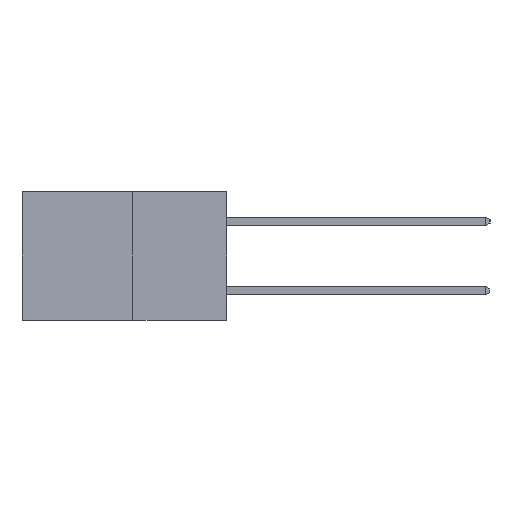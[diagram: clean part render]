
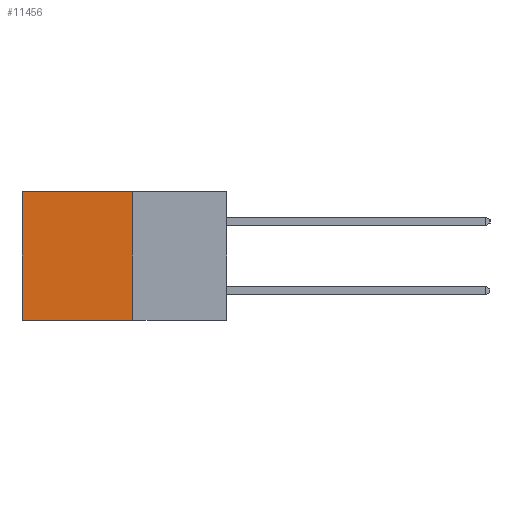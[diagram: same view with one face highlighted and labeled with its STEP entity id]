
A CAD part, left-side view. The second image highlights one B-rep face of the part: STEP entity #11456.
In plain terms, the highlighted planar face has unit normal (-1, 0, 0).
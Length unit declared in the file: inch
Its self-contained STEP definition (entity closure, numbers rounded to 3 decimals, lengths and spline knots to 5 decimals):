
#144 = LINE ( 'NONE', #14034, #7652 ) ;
#267 = EDGE_CURVE ( 'NONE', #5289, #16820, #5860, .T. ) ;
#419 = CARTESIAN_POINT ( 'NONE',  ( 0.277, 0.27, 0. ) ) ;
#1149 = DIRECTION ( 'NONE',  ( 0., 1., 0. ) ) ;
#1166 = CARTESIAN_POINT ( 'NONE',  ( 0.277, 0.27, 0. ) ) ;
#2502 = DIRECTION ( 'NONE',  ( 0., 0., -1. ) ) ;
#2637 = CARTESIAN_POINT ( 'NONE',  ( 0.277, 0.27, -0.37 ) ) ;
#2943 = EDGE_LOOP ( 'NONE', ( #11255, #3657, #3782, #6845 ) ) ;
#3618 = DIRECTION ( 'NONE',  ( 0., 0., -1. ) ) ;
#3657 = ORIENTED_EDGE ( 'NONE', *, *, #11526, .F. ) ;
#3782 = ORIENTED_EDGE ( 'NONE', *, *, #267, .F. ) ;
#4206 = CARTESIAN_POINT ( 'NONE',  ( 0.277, 0.59, -0.37 ) ) ;
#4404 = CARTESIAN_POINT ( 'NONE',  ( 0.277, 0.59, 0. ) ) ;
#4520 = AXIS2_PLACEMENT_3D ( 'NONE', #15528, #6944, #16915 ) ;
#4812 = VECTOR ( 'NONE', #11388, 39.37008 ) ;
#5289 = VERTEX_POINT ( 'NONE', #419 ) ;
#5518 = PLANE ( 'NONE',  #4520 ) ;
#5860 = LINE ( 'NONE', #2637, #6314 ) ;
#6314 = VECTOR ( 'NONE', #3618, 39.37008 ) ;
#6498 = EDGE_CURVE ( 'NONE', #5289, #6593, #15767, .T. ) ;
#6593 = VERTEX_POINT ( 'NONE', #4404 ) ;
#6845 = ORIENTED_EDGE ( 'NONE', *, *, #6498, .T. ) ;
#6944 = DIRECTION ( 'NONE',  ( 1., 0., 0. ) ) ;
#7652 = VECTOR ( 'NONE', #2502, 39.37008 ) ;
#8484 = CARTESIAN_POINT ( 'NONE',  ( 0.277, 0.27, -0.37 ) ) ;
#9959 = VECTOR ( 'NONE', #1149, 39.37008 ) ;
#10420 = LINE ( 'NONE', #8484, #9959 ) ;
#11255 = ORIENTED_EDGE ( 'NONE', *, *, #14261, .T. ) ;
#11388 = DIRECTION ( 'NONE',  ( 0., 1., 0. ) ) ;
#11456 = ADVANCED_FACE ( 'NONE', ( #14253 ), #5518, .F. ) ;
#11526 = EDGE_CURVE ( 'NONE', #16820, #15602, #10420, .T. ) ;
#14034 = CARTESIAN_POINT ( 'NONE',  ( 0.277, 0.59, -0.37 ) ) ;
#14253 = FACE_OUTER_BOUND ( 'NONE', #2943, .T. ) ;
#14261 = EDGE_CURVE ( 'NONE', #6593, #15602, #144, .T. ) ;
#15528 = CARTESIAN_POINT ( 'NONE',  ( 0.277, 0.27, -0.37 ) ) ;
#15602 = VERTEX_POINT ( 'NONE', #4206 ) ;
#15651 = CARTESIAN_POINT ( 'NONE',  ( 0.277, 0.27, -0.37 ) ) ;
#15767 = LINE ( 'NONE', #1166, #4812 ) ;
#16820 = VERTEX_POINT ( 'NONE', #15651 ) ;
#16915 = DIRECTION ( 'NONE',  ( 0., 0., -1. ) ) ;
